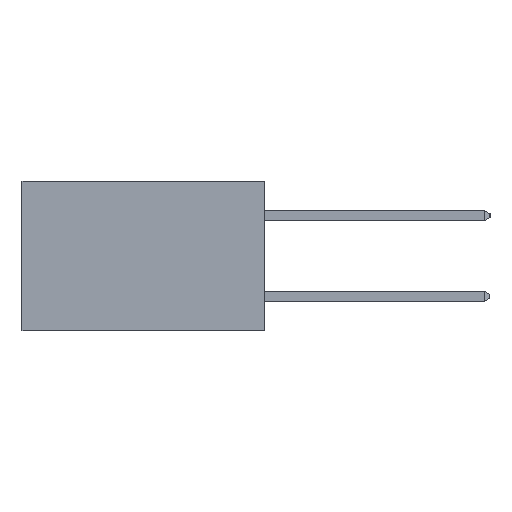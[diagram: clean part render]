
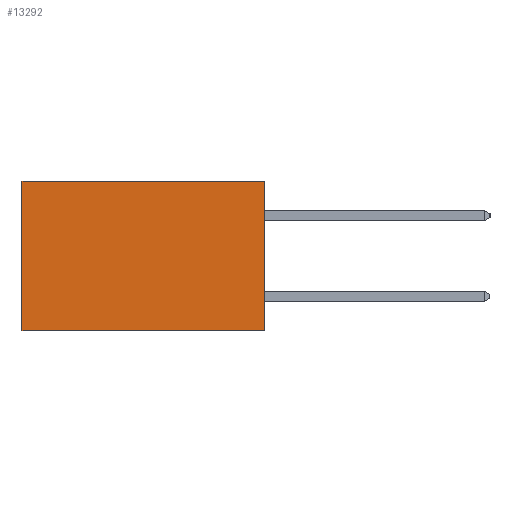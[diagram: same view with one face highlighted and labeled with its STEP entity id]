
A CAD part, left-side view. The second image highlights one B-rep face of the part: STEP entity #13292.
In plain terms, the highlighted planar face has unit normal (-1, 0, 0).
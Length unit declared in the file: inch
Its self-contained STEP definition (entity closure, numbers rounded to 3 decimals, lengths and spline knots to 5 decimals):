
#528 = DIRECTION ( 'NONE',  ( 0., 0., -1. ) ) ;
#1316 = CARTESIAN_POINT ( 'NONE',  ( 0.2615, 0., -0.37 ) ) ;
#1333 = EDGE_CURVE ( 'NONE', #4094, #4268, #9407, .T. ) ;
#1481 = VECTOR ( 'NONE', #10855, 39.37008 ) ;
#1581 = VECTOR ( 'NONE', #4230, 39.37008 ) ;
#2810 = LINE ( 'NONE', #17740, #1581 ) ;
#2832 = ORIENTED_EDGE ( 'NONE', *, *, #6963, .F. ) ;
#4094 = VERTEX_POINT ( 'NONE', #17872 ) ;
#4230 = DIRECTION ( 'NONE',  ( 0., 1., 0. ) ) ;
#4268 = VERTEX_POINT ( 'NONE', #7204 ) ;
#6281 = DIRECTION ( 'NONE',  ( 1., 0., 0. ) ) ;
#6901 = EDGE_CURVE ( 'NONE', #4094, #13374, #19692, .T. ) ;
#6963 = EDGE_CURVE ( 'NONE', #4268, #11741, #2810, .T. ) ;
#7204 = CARTESIAN_POINT ( 'NONE',  ( 0.2615, 0., -0.37 ) ) ;
#8834 = PLANE ( 'NONE',  #21105 ) ;
#8944 = CARTESIAN_POINT ( 'NONE',  ( 0.2615, 0.6, 0. ) ) ;
#9163 = ORIENTED_EDGE ( 'NONE', *, *, #14778, .T. ) ;
#9407 = LINE ( 'NONE', #1316, #10496 ) ;
#10496 = VECTOR ( 'NONE', #21504, 39.37008 ) ;
#10536 = LINE ( 'NONE', #17240, #1481 ) ;
#10855 = DIRECTION ( 'NONE',  ( 0., 0., -1. ) ) ;
#11365 = VECTOR ( 'NONE', #13322, 39.37008 ) ;
#11741 = VERTEX_POINT ( 'NONE', #19703 ) ;
#12463 = CARTESIAN_POINT ( 'NONE',  ( 0.2615, 0., -0.37 ) ) ;
#13292 = ADVANCED_FACE ( 'NONE', ( #21320 ), #8834, .F. ) ;
#13322 = DIRECTION ( 'NONE',  ( 0., 1., 0. ) ) ;
#13374 = VERTEX_POINT ( 'NONE', #8944 ) ;
#14778 = EDGE_CURVE ( 'NONE', #13374, #11741, #10536, .T. ) ;
#17240 = CARTESIAN_POINT ( 'NONE',  ( 0.2615, 0.6, -0.37 ) ) ;
#17285 = ORIENTED_EDGE ( 'NONE', *, *, #1333, .F. ) ;
#17740 = CARTESIAN_POINT ( 'NONE',  ( 0.2615, 0., -0.37 ) ) ;
#17800 = ORIENTED_EDGE ( 'NONE', *, *, #6901, .T. ) ;
#17808 = EDGE_LOOP ( 'NONE', ( #9163, #2832, #17285, #17800 ) ) ;
#17872 = CARTESIAN_POINT ( 'NONE',  ( 0.2615, 0., 0. ) ) ;
#19692 = LINE ( 'NONE', #21330, #11365 ) ;
#19703 = CARTESIAN_POINT ( 'NONE',  ( 0.2615, 0.6, -0.37 ) ) ;
#21105 = AXIS2_PLACEMENT_3D ( 'NONE', #12463, #6281, #528 ) ;
#21320 = FACE_OUTER_BOUND ( 'NONE', #17808, .T. ) ;
#21330 = CARTESIAN_POINT ( 'NONE',  ( 0.2615, 0., 0. ) ) ;
#21504 = DIRECTION ( 'NONE',  ( 0., 0., -1. ) ) ;
